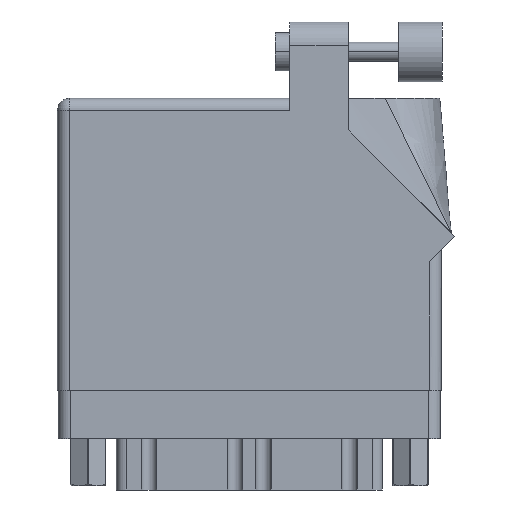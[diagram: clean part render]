
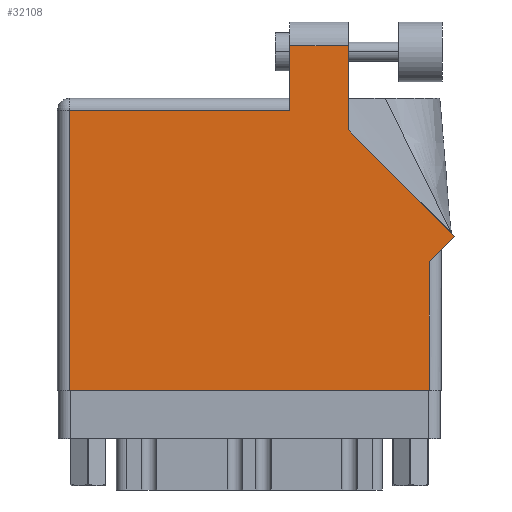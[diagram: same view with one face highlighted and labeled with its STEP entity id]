
A CAD part, front view. The second image highlights one B-rep face of the part: STEP entity #32108.
In plain terms, the highlighted face is planar.
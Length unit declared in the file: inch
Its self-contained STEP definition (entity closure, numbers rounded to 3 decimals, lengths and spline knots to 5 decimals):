
#1520 = LINE ( 'NONE', #5037, #14408 ) ;
#1699 = ORIENTED_EDGE ( 'NONE', *, *, #36809, .T. ) ;
#1739 = CARTESIAN_POINT ( 'NONE',  ( 1.524, 1.36442, 0. ) ) ;
#2926 = LINE ( 'NONE', #40221, #35651 ) ;
#3471 = ORIENTED_EDGE ( 'NONE', *, *, #35080, .T. ) ;
#5037 = CARTESIAN_POINT ( 'NONE',  ( 2.01, 0.737, 0. ) ) ;
#5419 = ORIENTED_EDGE ( 'NONE', *, *, #11806, .T. ) ;
#5421 = LINE ( 'NONE', #14901, #39937 ) ;
#6198 = AXIS2_PLACEMENT_3D ( 'NONE', #29268, #18669, #18449 ) ;
#6488 = LINE ( 'NONE', #12868, #36466 ) ;
#6807 = CARTESIAN_POINT ( 'NONE',  ( 1.524, 1.805, 0. ) ) ;
#8108 = VERTEX_POINT ( 'NONE', #29797 ) ;
#8704 = EDGE_CURVE ( 'NONE', #8108, #18057, #21525, .T. ) ;
#10010 = VERTEX_POINT ( 'NONE', #1739 ) ;
#11268 = LINE ( 'NONE', #20775, #36795 ) ;
#11806 = EDGE_CURVE ( 'NONE', #36937, #10010, #11268, .T. ) ;
#12868 = CARTESIAN_POINT ( 'NONE',  ( 1.524, 1.36442, 0. ) ) ;
#13582 = ORIENTED_EDGE ( 'NONE', *, *, #8704, .T. ) ;
#14049 = EDGE_CURVE ( 'NONE', #24597, #41434, #26128, .T. ) ;
#14408 = VECTOR ( 'NONE', #41883, 39.37008 ) ;
#14901 = CARTESIAN_POINT ( 'NONE',  ( 1.948, 0.737, 0. ) ) ;
#15331 = EDGE_CURVE ( 'NONE', #10010, #35406, #6488, .T. ) ;
#15777 = FACE_OUTER_BOUND ( 'NONE', #32704, .T. ) ;
#15833 = LINE ( 'NONE', #25565, #34361 ) ;
#15954 = DIRECTION ( 'NONE',  ( 1., 0., 0. ) ) ;
#16645 = VECTOR ( 'NONE', #15954, 39.37008 ) ;
#17807 = ORIENTED_EDGE ( 'NONE', *, *, #26209, .T. ) ;
#17910 = VECTOR ( 'NONE', #40388, 39.37008 ) ;
#18057 = VERTEX_POINT ( 'NONE', #41109 ) ;
#18449 = DIRECTION ( 'NONE',  ( -1., 0., 0. ) ) ;
#18669 = DIRECTION ( 'NONE',  ( 0., 0., -1. ) ) ;
#19321 = VECTOR ( 'NONE', #23996, 39.37008 ) ;
#19344 = ORIENTED_EDGE ( 'NONE', *, *, #37449, .T. ) ;
#20172 = CARTESIAN_POINT ( 'NONE',  ( 0., 0., 0. ) ) ;
#20337 = LINE ( 'NONE', #26957, #17910 ) ;
#20775 = CARTESIAN_POINT ( 'NONE',  ( 2.08071, 0.80771, 0. ) ) ;
#21525 = LINE ( 'NONE', #27966, #19321 ) ;
#21755 = DIRECTION ( 'NONE',  ( 0., 1., 0. ) ) ;
#23996 = DIRECTION ( 'NONE',  ( 0., -1., 0. ) ) ;
#24597 = VERTEX_POINT ( 'NONE', #41103 ) ;
#24653 = ORIENTED_EDGE ( 'NONE', *, *, #15331, .T. ) ;
#25565 = CARTESIAN_POINT ( 'NONE',  ( 1.217, 1.805, 0. ) ) ;
#26128 = LINE ( 'NONE', #20172, #16645 ) ;
#26209 = EDGE_CURVE ( 'NONE', #18057, #38978, #20337, .T. ) ;
#26957 = CARTESIAN_POINT ( 'NONE',  ( 0., 1.468, 0. ) ) ;
#26999 = DIRECTION ( 'NONE',  ( 0., -1., 0. ) ) ;
#27196 = DIRECTION ( 'NONE',  ( -0.707, 0.707, 0. ) ) ;
#27966 = CARTESIAN_POINT ( 'NONE',  ( 1.217, 1.53, 0. ) ) ;
#29268 = CARTESIAN_POINT ( 'NONE',  ( 0., 1.53, 0. ) ) ;
#29324 = DIRECTION ( 'NONE',  ( -1., 0., 0. ) ) ;
#29797 = CARTESIAN_POINT ( 'NONE',  ( 1.217, 1.805, 0. ) ) ;
#30124 = DIRECTION ( 'NONE',  ( 0., 1., 0. ) ) ;
#31613 = CARTESIAN_POINT ( 'NONE',  ( 1.948, 0., 0. ) ) ;
#31722 = EDGE_CURVE ( 'NONE', #35406, #8108, #15833, .T. ) ;
#32108 = ADVANCED_FACE ( 'NONE', ( #15777 ), #42477, .F. ) ;
#32704 = EDGE_LOOP ( 'NONE', ( #24653, #40521, #13582, #17807, #1699, #34388, #19344, #3471, #5419 ) ) ;
#33383 = CARTESIAN_POINT ( 'NONE',  ( 2.08071, 0.80771, 0. ) ) ;
#34361 = VECTOR ( 'NONE', #29324, 39.37008 ) ;
#34388 = ORIENTED_EDGE ( 'NONE', *, *, #14049, .T. ) ;
#35080 = EDGE_CURVE ( 'NONE', #41752, #36937, #1520, .T. ) ;
#35406 = VERTEX_POINT ( 'NONE', #6807 ) ;
#35651 = VECTOR ( 'NONE', #26999, 39.37008 ) ;
#36466 = VECTOR ( 'NONE', #30124, 39.37008 ) ;
#36795 = VECTOR ( 'NONE', #27196, 39.37008 ) ;
#36809 = EDGE_CURVE ( 'NONE', #38978, #24597, #2926, .T. ) ;
#36937 = VERTEX_POINT ( 'NONE', #33383 ) ;
#37449 = EDGE_CURVE ( 'NONE', #41434, #41752, #5421, .T. ) ;
#38147 = CARTESIAN_POINT ( 'NONE',  ( 1.948, 0.675, 0. ) ) ;
#38978 = VERTEX_POINT ( 'NONE', #39833 ) ;
#39833 = CARTESIAN_POINT ( 'NONE',  ( 0.062, 1.468, 0. ) ) ;
#39937 = VECTOR ( 'NONE', #21755, 39.37008 ) ;
#40221 = CARTESIAN_POINT ( 'NONE',  ( 0.062, 0., 0. ) ) ;
#40388 = DIRECTION ( 'NONE',  ( -1., 0., 0. ) ) ;
#40521 = ORIENTED_EDGE ( 'NONE', *, *, #31722, .T. ) ;
#41103 = CARTESIAN_POINT ( 'NONE',  ( 0.062, 0., 0. ) ) ;
#41109 = CARTESIAN_POINT ( 'NONE',  ( 1.217, 1.468, 0. ) ) ;
#41434 = VERTEX_POINT ( 'NONE', #31613 ) ;
#41752 = VERTEX_POINT ( 'NONE', #38147 ) ;
#41883 = DIRECTION ( 'NONE',  ( 0.707, 0.707, 0. ) ) ;
#42477 = PLANE ( 'NONE',  #6198 ) ;
